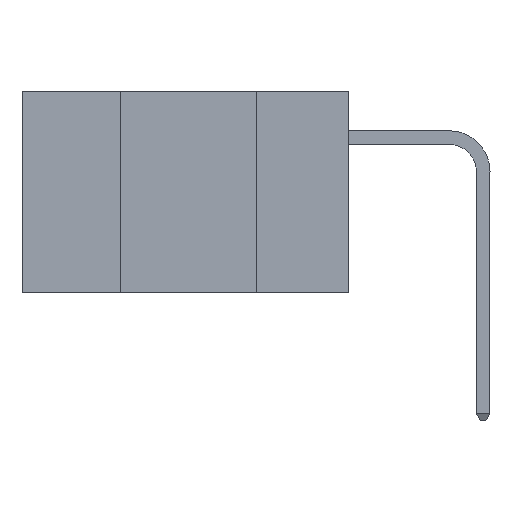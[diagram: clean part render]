
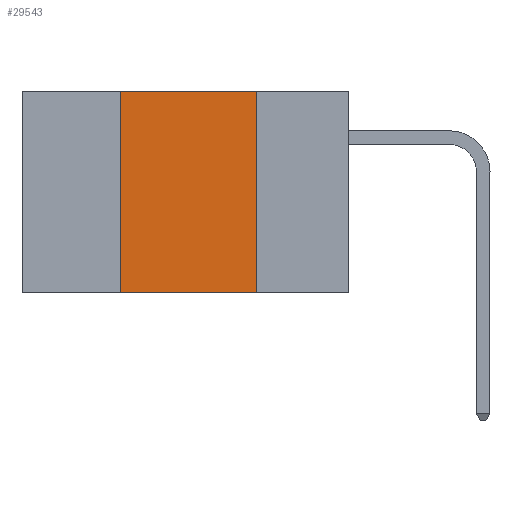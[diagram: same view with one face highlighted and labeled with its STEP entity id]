
A CAD part, left-side view. The second image highlights one B-rep face of the part: STEP entity #29543.
In plain terms, the highlighted planar face has unit normal (-1, 0, 0).
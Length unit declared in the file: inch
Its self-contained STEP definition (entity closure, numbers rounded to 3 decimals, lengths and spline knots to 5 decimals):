
#760 = DIRECTION ( 'NONE',  ( 0., 0., -1. ) ) ;
#3066 = LINE ( 'NONE', #12303, #25610 ) ;
#3089 = VERTEX_POINT ( 'NONE', #6465 ) ;
#5454 = LINE ( 'NONE', #16845, #13264 ) ;
#5547 = EDGE_CURVE ( 'NONE', #15172, #12724, #27874, .T. ) ;
#6465 = CARTESIAN_POINT ( 'NONE',  ( 0., 0.17, 0. ) ) ;
#7713 = ORIENTED_EDGE ( 'NONE', *, *, #8522, .T. ) ;
#8522 = EDGE_CURVE ( 'NONE', #15172, #9316, #5454, .T. ) ;
#9316 = VERTEX_POINT ( 'NONE', #23435 ) ;
#9450 = EDGE_CURVE ( 'NONE', #3089, #9316, #3066, .T. ) ;
#9754 = CARTESIAN_POINT ( 'NONE',  ( 0., 0.42, 0. ) ) ;
#11196 = CARTESIAN_POINT ( 'NONE',  ( 0., 0.42, -0.37 ) ) ;
#12303 = CARTESIAN_POINT ( 'NONE',  ( 0., 0.17, 0. ) ) ;
#12546 = PLANE ( 'NONE',  #13277 ) ;
#12724 = VERTEX_POINT ( 'NONE', #17766 ) ;
#13264 = VECTOR ( 'NONE', #37102, 39.37008 ) ;
#13277 = AXIS2_PLACEMENT_3D ( 'NONE', #24193, #18431, #760 ) ;
#15172 = VERTEX_POINT ( 'NONE', #11196 ) ;
#16211 = EDGE_CURVE ( 'NONE', #12724, #3089, #19034, .T. ) ;
#16845 = CARTESIAN_POINT ( 'NONE',  ( 0., 0.6, -0.37 ) ) ;
#17766 = CARTESIAN_POINT ( 'NONE',  ( 0., 0.42, 0. ) ) ;
#18122 = VECTOR ( 'NONE', #23441, 39.37008 ) ;
#18431 = DIRECTION ( 'NONE',  ( 1., 0., 0. ) ) ;
#19034 = LINE ( 'NONE', #20522, #18122 ) ;
#20522 = CARTESIAN_POINT ( 'NONE',  ( 0., 0.6, 0. ) ) ;
#23435 = CARTESIAN_POINT ( 'NONE',  ( 0., 0.17, -0.37 ) ) ;
#23441 = DIRECTION ( 'NONE',  ( 0., -1., 0. ) ) ;
#23961 = DIRECTION ( 'NONE',  ( 0., 0., -1. ) ) ;
#24193 = CARTESIAN_POINT ( 'NONE',  ( 0., 0.6, 0. ) ) ;
#24728 = EDGE_LOOP ( 'NONE', ( #34159, #27415, #30140, #7713 ) ) ;
#25610 = VECTOR ( 'NONE', #23961, 39.37008 ) ;
#27286 = DIRECTION ( 'NONE',  ( 0., 0., 1. ) ) ;
#27415 = ORIENTED_EDGE ( 'NONE', *, *, #16211, .F. ) ;
#27874 = LINE ( 'NONE', #9754, #35513 ) ;
#29543 = ADVANCED_FACE ( 'NONE', ( #36331 ), #12546, .F. ) ;
#30140 = ORIENTED_EDGE ( 'NONE', *, *, #5547, .F. ) ;
#34159 = ORIENTED_EDGE ( 'NONE', *, *, #9450, .F. ) ;
#35513 = VECTOR ( 'NONE', #27286, 39.37008 ) ;
#36331 = FACE_OUTER_BOUND ( 'NONE', #24728, .T. ) ;
#37102 = DIRECTION ( 'NONE',  ( 0., -1., 0. ) ) ;
